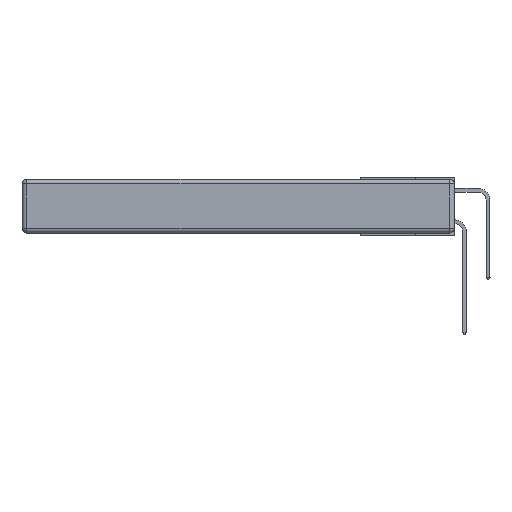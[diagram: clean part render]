
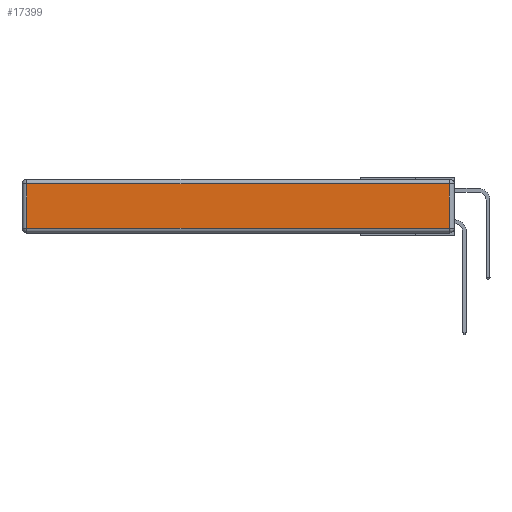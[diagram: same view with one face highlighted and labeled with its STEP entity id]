
A CAD part, left-side view. The second image highlights one B-rep face of the part: STEP entity #17399.
In plain terms, the highlighted planar face has unit normal (-1, 0, 0).
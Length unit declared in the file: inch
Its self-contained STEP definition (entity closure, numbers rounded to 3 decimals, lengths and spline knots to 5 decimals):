
#388 = EDGE_LOOP ( 'NONE', ( #651, #11885, #8376, #7839 ) ) ;
#562 = VERTEX_POINT ( 'NONE', #9461 ) ;
#651 = ORIENTED_EDGE ( 'NONE', *, *, #8682, .T. ) ;
#1326 = EDGE_CURVE ( 'NONE', #562, #15948, #11040, .T. ) ;
#1452 = CARTESIAN_POINT ( 'NONE',  ( 0., 0.03, -0.313 ) ) ;
#2064 = AXIS2_PLACEMENT_3D ( 'NONE', #8753, #11121, #12350 ) ;
#2726 = DIRECTION ( 'NONE',  ( 0., 0., 1. ) ) ;
#2978 = VECTOR ( 'NONE', #2726, 39.37008 ) ;
#3117 = PLANE ( 'NONE',  #2064 ) ;
#5882 = CARTESIAN_POINT ( 'NONE',  ( 0., 2.72, -0.313 ) ) ;
#5907 = CARTESIAN_POINT ( 'NONE',  ( 0., 2.75, -0.03 ) ) ;
#6004 = EDGE_CURVE ( 'NONE', #11656, #8514, #18267, .T. ) ;
#7221 = LINE ( 'NONE', #7687, #8564 ) ;
#7322 = CARTESIAN_POINT ( 'NONE',  ( 0., 2.72, -0.343 ) ) ;
#7624 = VECTOR ( 'NONE', #17536, 39.37008 ) ;
#7687 = CARTESIAN_POINT ( 'NONE',  ( 0., 0., -0.313 ) ) ;
#7839 = ORIENTED_EDGE ( 'NONE', *, *, #1326, .T. ) ;
#8376 = ORIENTED_EDGE ( 'NONE', *, *, #10152, .T. ) ;
#8514 = VERTEX_POINT ( 'NONE', #9445 ) ;
#8564 = VECTOR ( 'NONE', #9009, 39.37008 ) ;
#8682 = EDGE_CURVE ( 'NONE', #15948, #11656, #7221, .T. ) ;
#8753 = CARTESIAN_POINT ( 'NONE',  ( 0., 0., -0.343 ) ) ;
#9009 = DIRECTION ( 'NONE',  ( 0., -1., 0. ) ) ;
#9445 = CARTESIAN_POINT ( 'NONE',  ( 0., 0.03, -0.03 ) ) ;
#9461 = CARTESIAN_POINT ( 'NONE',  ( 0., 2.72, -0.03 ) ) ;
#10152 = EDGE_CURVE ( 'NONE', #8514, #562, #15179, .T. ) ;
#11040 = LINE ( 'NONE', #7322, #16820 ) ;
#11121 = DIRECTION ( 'NONE',  ( -1., 0., 0. ) ) ;
#11656 = VERTEX_POINT ( 'NONE', #1452 ) ;
#11885 = ORIENTED_EDGE ( 'NONE', *, *, #6004, .T. ) ;
#12350 = DIRECTION ( 'NONE',  ( 0., 0., 1. ) ) ;
#15179 = LINE ( 'NONE', #5907, #7624 ) ;
#15496 = CARTESIAN_POINT ( 'NONE',  ( 0., 0.03, -0.343 ) ) ;
#15571 = FACE_OUTER_BOUND ( 'NONE', #388, .T. ) ;
#15948 = VERTEX_POINT ( 'NONE', #5882 ) ;
#16820 = VECTOR ( 'NONE', #17475, 39.37008 ) ;
#17399 = ADVANCED_FACE ( 'NONE', ( #15571 ), #3117, .T. ) ;
#17475 = DIRECTION ( 'NONE',  ( 0., 0., -1. ) ) ;
#17536 = DIRECTION ( 'NONE',  ( 0., 1., 0. ) ) ;
#18267 = LINE ( 'NONE', #15496, #2978 ) ;
